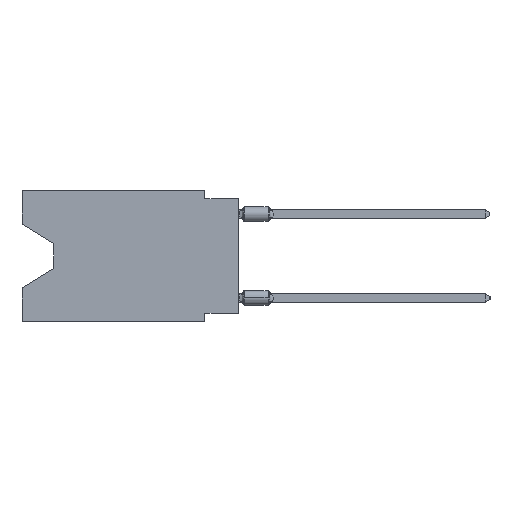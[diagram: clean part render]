
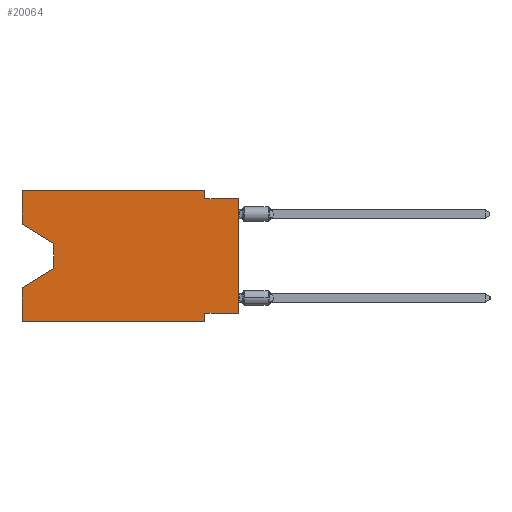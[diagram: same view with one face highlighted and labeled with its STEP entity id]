
A CAD part, left-side view. The second image highlights one B-rep face of the part: STEP entity #20064.
In plain terms, the highlighted planar face has unit normal (-1, 0, 0).
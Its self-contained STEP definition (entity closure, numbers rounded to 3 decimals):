
#32 = ORIENTED_EDGE ( 'NONE', *, *, #8615, .F. ) ;
#134 = VECTOR ( 'NONE', #46902, 1000. ) ;
#545 = CARTESIAN_POINT ( 'NONE',  ( 0., 0., 0. ) ) ;
#558 = CARTESIAN_POINT ( 'NONE',  ( 0., 2.54, -0.635 ) ) ;
#1800 = CARTESIAN_POINT ( 'NONE',  ( 0., 16.383, -2.546 ) ) ;
#1862 = CARTESIAN_POINT ( 'NONE',  ( 0., 2.54, -9.271 ) ) ;
#3085 = CARTESIAN_POINT ( 'NONE',  ( 0., 13.97, -5.893 ) ) ;
#4187 = CARTESIAN_POINT ( 'NONE',  ( 0., 13.97, -4.013 ) ) ;
#4197 = DIRECTION ( 'NONE',  ( 0., -0.855, -0.519 ) ) ;
#4390 = LINE ( 'NONE', #38160, #22702 ) ;
#4796 = EDGE_CURVE ( 'NONE', #41109, #38506, #27197, .T. ) ;
#5484 = VECTOR ( 'NONE', #26265, 1000. ) ;
#6245 = VERTEX_POINT ( 'NONE', #8992 ) ;
#6264 = PLANE ( 'NONE',  #45408 ) ;
#7101 = LINE ( 'NONE', #18750, #30268 ) ;
#7166 = VECTOR ( 'NONE', #34527, 1000. ) ;
#7248 = VECTOR ( 'NONE', #19844, 1000. ) ;
#7350 = VERTEX_POINT ( 'NONE', #35184 ) ;
#7480 = CARTESIAN_POINT ( 'NONE',  ( 0., 16.383, -9.906 ) ) ;
#8317 = LINE ( 'NONE', #33354, #10278 ) ;
#8615 = EDGE_CURVE ( 'NONE', #21015, #7350, #25642, .T. ) ;
#8992 = CARTESIAN_POINT ( 'NONE',  ( 0., 16.383, -7.36 ) ) ;
#9015 = DIRECTION ( 'NONE',  ( 0., 0., 1. ) ) ;
#9955 = VERTEX_POINT ( 'NONE', #3085 ) ;
#10136 = DIRECTION ( 'NONE',  ( 0., 0., -1. ) ) ;
#10278 = VECTOR ( 'NONE', #11457, 1000. ) ;
#10356 = ORIENTED_EDGE ( 'NONE', *, *, #13430, .F. ) ;
#10535 = VERTEX_POINT ( 'NONE', #1800 ) ;
#10660 = VECTOR ( 'NONE', #36371, 1000. ) ;
#10821 = EDGE_CURVE ( 'NONE', #11203, #9955, #30392, .T. ) ;
#11203 = VERTEX_POINT ( 'NONE', #36478 ) ;
#11457 = DIRECTION ( 'NONE',  ( 0., 0., -1. ) ) ;
#11857 = LINE ( 'NONE', #37419, #23682 ) ;
#12122 = CARTESIAN_POINT ( 'NONE',  ( 0., 16.383, 0. ) ) ;
#12642 = LINE ( 'NONE', #545, #36126 ) ;
#12742 = CARTESIAN_POINT ( 'NONE',  ( 0., 2.54, -9.906 ) ) ;
#13333 = CARTESIAN_POINT ( 'NONE',  ( 0., 13.97, -5.893 ) ) ;
#13430 = EDGE_CURVE ( 'NONE', #15538, #6245, #16388, .T. ) ;
#13859 = EDGE_CURVE ( 'NONE', #9955, #6245, #17226, .T. ) ;
#15538 = VERTEX_POINT ( 'NONE', #7480 ) ;
#15646 = ORIENTED_EDGE ( 'NONE', *, *, #10821, .T. ) ;
#15944 = CARTESIAN_POINT ( 'NONE',  ( 0., 0., -0.635 ) ) ;
#16011 = ORIENTED_EDGE ( 'NONE', *, *, #27535, .T. ) ;
#16388 = LINE ( 'NONE', #31940, #28014 ) ;
#17172 = ORIENTED_EDGE ( 'NONE', *, *, #13859, .T. ) ;
#17226 = LINE ( 'NONE', #13333, #134 ) ;
#18673 = DIRECTION ( 'NONE',  ( 0., -1., 0. ) ) ;
#18750 = CARTESIAN_POINT ( 'NONE',  ( 0., 16.383, -2.546 ) ) ;
#19346 = LINE ( 'NONE', #15944, #7248 ) ;
#19844 = DIRECTION ( 'NONE',  ( 0., -1., 0. ) ) ;
#20064 = ADVANCED_FACE ( 'NONE', ( #20640 ), #6264, .F. ) ;
#20640 = FACE_OUTER_BOUND ( 'NONE', #34552, .T. ) ;
#20674 = VERTEX_POINT ( 'NONE', #558 ) ;
#21015 = VERTEX_POINT ( 'NONE', #12122 ) ;
#22302 = EDGE_CURVE ( 'NONE', #38506, #47552, #4390, .T. ) ;
#22702 = VECTOR ( 'NONE', #34263, 1000. ) ;
#23682 = VECTOR ( 'NONE', #18673, 1000. ) ;
#23779 = ORIENTED_EDGE ( 'NONE', *, *, #22302, .F. ) ;
#24819 = EDGE_CURVE ( 'NONE', #7350, #20674, #8317, .T. ) ;
#25642 = LINE ( 'NONE', #33425, #10660 ) ;
#26265 = DIRECTION ( 'NONE',  ( 0., 0., -1. ) ) ;
#27197 = LINE ( 'NONE', #44960, #7166 ) ;
#27535 = EDGE_CURVE ( 'NONE', #41109, #35461, #12642, .T. ) ;
#28014 = VECTOR ( 'NONE', #38553, 1000. ) ;
#28683 = EDGE_CURVE ( 'NONE', #10535, #11203, #7101, .T. ) ;
#30268 = VECTOR ( 'NONE', #4197, 1000. ) ;
#30392 = LINE ( 'NONE', #4187, #5484 ) ;
#31940 = CARTESIAN_POINT ( 'NONE',  ( 0., 16.383, 0. ) ) ;
#32405 = EDGE_CURVE ( 'NONE', #20674, #35461, #19346, .T. ) ;
#33060 = ORIENTED_EDGE ( 'NONE', *, *, #42135, .T. ) ;
#33354 = CARTESIAN_POINT ( 'NONE',  ( 0., 2.54, 0. ) ) ;
#33425 = CARTESIAN_POINT ( 'NONE',  ( 0., 16.383, 0. ) ) ;
#34263 = DIRECTION ( 'NONE',  ( 0., 0., -1. ) ) ;
#34527 = DIRECTION ( 'NONE',  ( 0., 1., 0. ) ) ;
#34552 = EDGE_LOOP ( 'NONE', ( #45171, #15646, #17172, #10356, #33060, #23779, #35550, #16011, #36043, #43661, #32, #47300 ) ) ;
#35184 = CARTESIAN_POINT ( 'NONE',  ( 0., 2.54, 0. ) ) ;
#35461 = VERTEX_POINT ( 'NONE', #42169 ) ;
#35550 = ORIENTED_EDGE ( 'NONE', *, *, #4796, .F. ) ;
#35718 = LINE ( 'NONE', #42550, #42439 ) ;
#35837 = CARTESIAN_POINT ( 'NONE',  ( 0., 0., -9.271 ) ) ;
#36043 = ORIENTED_EDGE ( 'NONE', *, *, #32405, .F. ) ;
#36126 = VECTOR ( 'NONE', #9015, 1000. ) ;
#36371 = DIRECTION ( 'NONE',  ( 0., -1., 0. ) ) ;
#36478 = CARTESIAN_POINT ( 'NONE',  ( 0., 13.97, -4.013 ) ) ;
#37419 = CARTESIAN_POINT ( 'NONE',  ( 0., 16.383, -9.906 ) ) ;
#38160 = CARTESIAN_POINT ( 'NONE',  ( 0., 2.54, -9.906 ) ) ;
#38506 = VERTEX_POINT ( 'NONE', #1862 ) ;
#38553 = DIRECTION ( 'NONE',  ( 0., 0., 1. ) ) ;
#39118 = DIRECTION ( 'NONE',  ( 1., 0., 0. ) ) ;
#41109 = VERTEX_POINT ( 'NONE', #35837 ) ;
#42135 = EDGE_CURVE ( 'NONE', #15538, #47552, #11857, .T. ) ;
#42169 = CARTESIAN_POINT ( 'NONE',  ( 0., 0., -0.635 ) ) ;
#42439 = VECTOR ( 'NONE', #42777, 1000. ) ;
#42550 = CARTESIAN_POINT ( 'NONE',  ( 0., 16.383, 0. ) ) ;
#42777 = DIRECTION ( 'NONE',  ( 0., 0., 1. ) ) ;
#43519 = EDGE_CURVE ( 'NONE', #10535, #21015, #35718, .T. ) ;
#43661 = ORIENTED_EDGE ( 'NONE', *, *, #24819, .F. ) ;
#44960 = CARTESIAN_POINT ( 'NONE',  ( 0., 0., -9.271 ) ) ;
#45171 = ORIENTED_EDGE ( 'NONE', *, *, #28683, .T. ) ;
#45408 = AXIS2_PLACEMENT_3D ( 'NONE', #46624, #39118, #10136 ) ;
#46624 = CARTESIAN_POINT ( 'NONE',  ( 0., 16.383, 0. ) ) ;
#46902 = DIRECTION ( 'NONE',  ( 0., 0.855, -0.519 ) ) ;
#47300 = ORIENTED_EDGE ( 'NONE', *, *, #43519, .F. ) ;
#47552 = VERTEX_POINT ( 'NONE', #12742 ) ;
